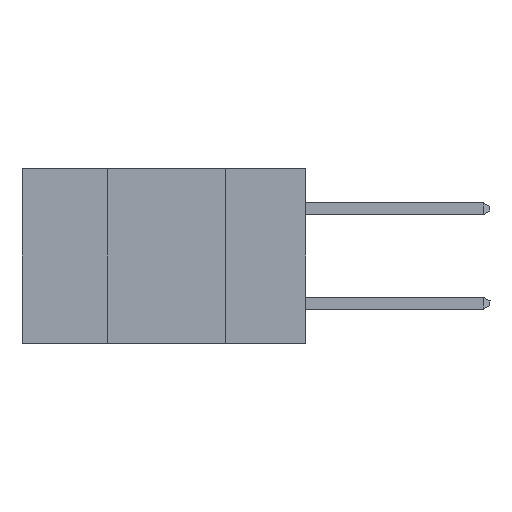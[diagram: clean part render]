
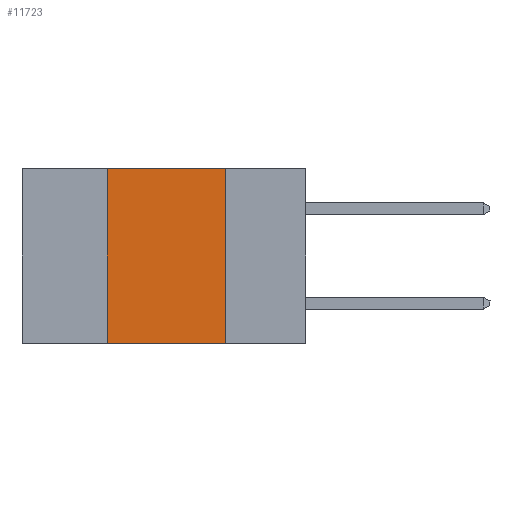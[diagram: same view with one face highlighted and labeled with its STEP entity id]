
A CAD part, left-side view. The second image highlights one B-rep face of the part: STEP entity #11723.
In plain terms, the highlighted planar face has unit normal (-1, 0, 0).
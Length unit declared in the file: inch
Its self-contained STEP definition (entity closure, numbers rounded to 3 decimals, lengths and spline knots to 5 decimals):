
#28 = CARTESIAN_POINT ( 'NONE',  ( 0., 0.17, 0. ) ) ;
#72 = DIRECTION ( 'NONE',  ( 0., 0., -1. ) ) ;
#111 = CARTESIAN_POINT ( 'NONE',  ( 0., 0.6, 0. ) ) ;
#1029 = CARTESIAN_POINT ( 'NONE',  ( 0., 0.6, 0. ) ) ;
#1092 = DIRECTION ( 'NONE',  ( 0., -1., 0. ) ) ;
#1461 = AXIS2_PLACEMENT_3D ( 'NONE', #1029, #7839, #8905 ) ;
#1631 = VECTOR ( 'NONE', #9334, 39.37008 ) ;
#2126 = CARTESIAN_POINT ( 'NONE',  ( 0., 0.42, 0. ) ) ;
#2186 = LINE ( 'NONE', #28, #9467 ) ;
#2536 = FACE_OUTER_BOUND ( 'NONE', #9991, .T. ) ;
#3042 = EDGE_CURVE ( 'NONE', #7292, #5828, #9367, .T. ) ;
#3527 = ORIENTED_EDGE ( 'NONE', *, *, #5580, .F. ) ;
#3594 = VERTEX_POINT ( 'NONE', #9987 ) ;
#4214 = ORIENTED_EDGE ( 'NONE', *, *, #5651, .F. ) ;
#5230 = VECTOR ( 'NONE', #1092, 39.37008 ) ;
#5406 = CARTESIAN_POINT ( 'NONE',  ( 0., 0.6, -0.37 ) ) ;
#5580 = EDGE_CURVE ( 'NONE', #3594, #5828, #2186, .T. ) ;
#5651 = EDGE_CURVE ( 'NONE', #8136, #3594, #7521, .T. ) ;
#5694 = LINE ( 'NONE', #6005, #10383 ) ;
#5828 = VERTEX_POINT ( 'NONE', #6421 ) ;
#6005 = CARTESIAN_POINT ( 'NONE',  ( 0., 0.42, 0. ) ) ;
#6209 = EDGE_CURVE ( 'NONE', #7292, #8136, #5694, .T. ) ;
#6421 = CARTESIAN_POINT ( 'NONE',  ( 0., 0.17, -0.37 ) ) ;
#6843 = PLANE ( 'NONE',  #1461 ) ;
#7292 = VERTEX_POINT ( 'NONE', #11161 ) ;
#7521 = LINE ( 'NONE', #111, #5230 ) ;
#7839 = DIRECTION ( 'NONE',  ( 1., 0., 0. ) ) ;
#7916 = DIRECTION ( 'NONE',  ( 0., 0., 1. ) ) ;
#7967 = ORIENTED_EDGE ( 'NONE', *, *, #3042, .T. ) ;
#8136 = VERTEX_POINT ( 'NONE', #2126 ) ;
#8905 = DIRECTION ( 'NONE',  ( 0., 0., -1. ) ) ;
#9334 = DIRECTION ( 'NONE',  ( 0., -1., 0. ) ) ;
#9367 = LINE ( 'NONE', #5406, #1631 ) ;
#9467 = VECTOR ( 'NONE', #72, 39.37008 ) ;
#9987 = CARTESIAN_POINT ( 'NONE',  ( 0., 0.17, 0. ) ) ;
#9991 = EDGE_LOOP ( 'NONE', ( #3527, #4214, #12100, #7967 ) ) ;
#10383 = VECTOR ( 'NONE', #7916, 39.37008 ) ;
#11161 = CARTESIAN_POINT ( 'NONE',  ( 0., 0.42, -0.37 ) ) ;
#11723 = ADVANCED_FACE ( 'NONE', ( #2536 ), #6843, .F. ) ;
#12100 = ORIENTED_EDGE ( 'NONE', *, *, #6209, .F. ) ;
